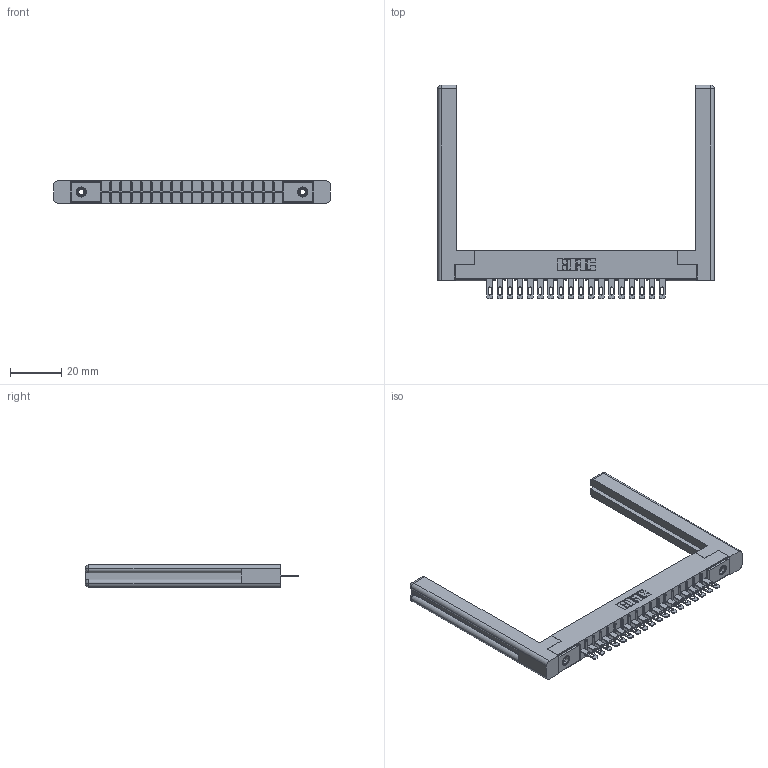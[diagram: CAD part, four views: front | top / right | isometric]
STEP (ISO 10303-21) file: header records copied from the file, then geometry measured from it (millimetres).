
FILE_DESCRIPTION (( 'STEP AP203' ), '1' );
FILE_NAME ('356-018-400-158.STEP', '2020-09-23T13:23:37', ( '' ), ( '' ), 'SwSTEP 2.0', 'SolidWorks 2020', '' );
FILE_SCHEMA (( 'CONFIG_CONTROL_DESIGN' ));
Length unit declared in the file: inch
Products named in the file (5): 356-018-400-158; 345-250-001_345-250-001-102; 306 Part_.156 Dia; 307-220-058; 306-290-001_100
Assembly tree (23 placements, depth 2):
  356-018-400-158
    306 Part_.156 Dia
    306-290-001_100  x18
    345-250-001_345-250-001-102  x2
    307-220-058  x2
Bounding box: 107.95 x 83.52 x 8.71 mm (x, y, z)
Volume: 15065.2 mm3; surface area: 16429.7 mm2
Topology: 23 solids, 23 shells, 1626 faces, 4540 edges, 2916 vertices
Faces by surface type: plane 1052, cylinder 478, sphere 72, cone 12, torus 12
Entity records: 22692 total; most frequent: CARTESIAN_POINT 3816, ORIENTED_EDGE 3722, DIRECTION 3721, EDGE_CURVE 1861, LINE 1435, VECTOR 1435, VERTEX_POINT 1184, AXIS2_PLACEMENT_3D 1143
